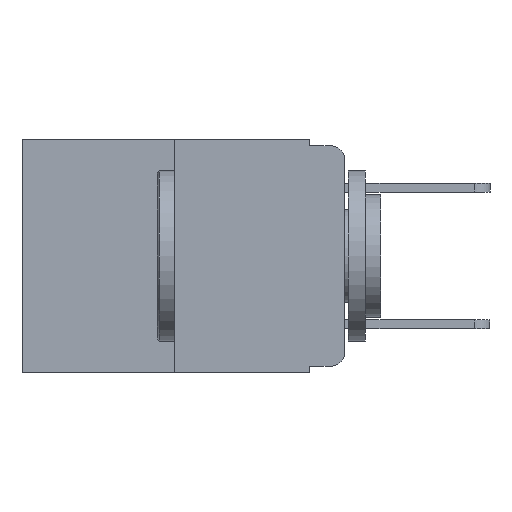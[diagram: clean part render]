
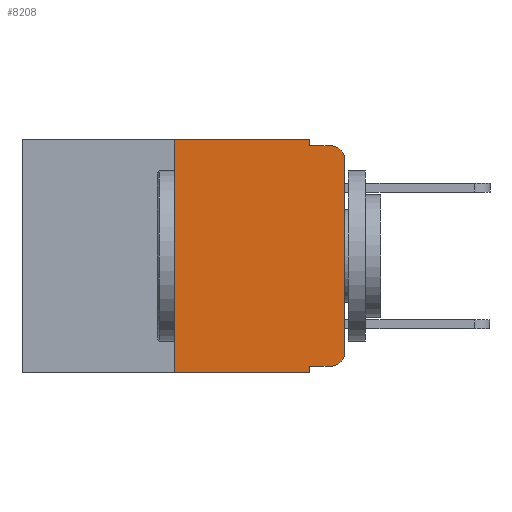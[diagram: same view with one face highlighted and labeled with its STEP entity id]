
A CAD part, left-side view. The second image highlights one B-rep face of the part: STEP entity #8208.
In plain terms, the highlighted planar face has unit normal (-1, 0, 0).
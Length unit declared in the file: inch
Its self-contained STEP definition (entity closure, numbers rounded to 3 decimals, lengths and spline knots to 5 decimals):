
#78 = ORIENTED_EDGE ( 'NONE', *, *, #8884, .T. ) ;
#179 = VECTOR ( 'NONE', #7538, 39.37008 ) ;
#377 = LINE ( 'NONE', #11194, #10634 ) ;
#400 = ORIENTED_EDGE ( 'NONE', *, *, #5301, .F. ) ;
#589 = VECTOR ( 'NONE', #1246, 39.37008 ) ;
#727 = ORIENTED_EDGE ( 'NONE', *, *, #4648, .F. ) ;
#831 = ORIENTED_EDGE ( 'NONE', *, *, #7722, .F. ) ;
#844 = VERTEX_POINT ( 'NONE', #8934 ) ;
#949 = CIRCLE ( 'NONE', #3947, 0.02 ) ;
#991 = LINE ( 'NONE', #10465, #589 ) ;
#995 = CARTESIAN_POINT ( 'NONE',  ( 0., 0.25, 0. ) ) ;
#1093 = VERTEX_POINT ( 'NONE', #7869 ) ;
#1246 = DIRECTION ( 'NONE',  ( 0., 0., -1. ) ) ;
#1350 = ORIENTED_EDGE ( 'NONE', *, *, #6838, .T. ) ;
#1418 = DIRECTION ( 'NONE',  ( 0., -1., 0. ) ) ;
#1528 = VECTOR ( 'NONE', #1418, 39.37008 ) ;
#1662 = ORIENTED_EDGE ( 'NONE', *, *, #7949, .F. ) ;
#1836 = CARTESIAN_POINT ( 'NONE',  ( 0., 0.25, -0.343 ) ) ;
#1956 = VERTEX_POINT ( 'NONE', #995 ) ;
#2018 = CIRCLE ( 'NONE', #9137, 0.02 ) ;
#2030 = VECTOR ( 'NONE', #7331, 39.37008 ) ;
#2068 = EDGE_CURVE ( 'NONE', #10869, #5049, #2018, .T. ) ;
#2095 = CARTESIAN_POINT ( 'NONE',  ( 0., 0.25, 0. ) ) ;
#2218 = DIRECTION ( 'NONE',  ( 0., 0., 1. ) ) ;
#2308 = VERTEX_POINT ( 'NONE', #6984 ) ;
#2338 = ORIENTED_EDGE ( 'NONE', *, *, #2068, .T. ) ;
#2448 = ORIENTED_EDGE ( 'NONE', *, *, #9439, .T. ) ;
#2637 = FACE_OUTER_BOUND ( 'NONE', #10825, .T. ) ;
#2736 = VERTEX_POINT ( 'NONE', #8588 ) ;
#2799 = CARTESIAN_POINT ( 'NONE',  ( 0., 0.051, 0. ) ) ;
#2853 = CARTESIAN_POINT ( 'NONE',  ( 0., 0.473, 0. ) ) ;
#3087 = VERTEX_POINT ( 'NONE', #5544 ) ;
#3395 = EDGE_CURVE ( 'NONE', #2736, #10869, #377, .T. ) ;
#3702 = CARTESIAN_POINT ( 'NONE',  ( 0., 0.02, -0.313 ) ) ;
#3719 = VERTEX_POINT ( 'NONE', #1836 ) ;
#3947 = AXIS2_PLACEMENT_3D ( 'NONE', #4903, #10981, #5855 ) ;
#4031 = EDGE_CURVE ( 'NONE', #2736, #2308, #991, .T. ) ;
#4080 = ORIENTED_EDGE ( 'NONE', *, *, #4031, .F. ) ;
#4096 = DIRECTION ( 'NONE',  ( 0., 0., -1. ) ) ;
#4201 = AXIS2_PLACEMENT_3D ( 'NONE', #11030, #4991, #11054 ) ;
#4255 = CARTESIAN_POINT ( 'NONE',  ( 0., 0.051, 0. ) ) ;
#4440 = VECTOR ( 'NONE', #2218, 39.37008 ) ;
#4560 = VECTOR ( 'NONE', #7439, 39.37008 ) ;
#4590 = LINE ( 'NONE', #6442, #2030 ) ;
#4648 = EDGE_CURVE ( 'NONE', #3719, #1956, #7183, .T. ) ;
#4903 = CARTESIAN_POINT ( 'NONE',  ( 0., 0.02, -0.03 ) ) ;
#4991 = DIRECTION ( 'NONE',  ( 1., 0., 0. ) ) ;
#5049 = VERTEX_POINT ( 'NONE', #5319 ) ;
#5301 = EDGE_CURVE ( 'NONE', #10631, #1093, #7029, .T. ) ;
#5319 = CARTESIAN_POINT ( 'NONE',  ( 0., 0., -0.313 ) ) ;
#5544 = CARTESIAN_POINT ( 'NONE',  ( 0., 0.02, -0.01 ) ) ;
#5660 = LINE ( 'NONE', #2853, #179 ) ;
#5855 = DIRECTION ( 'NONE',  ( 0., 0., -1. ) ) ;
#6178 = LINE ( 'NONE', #9025, #8261 ) ;
#6442 = CARTESIAN_POINT ( 'NONE',  ( 0., 0.051, -0.01 ) ) ;
#6838 = EDGE_CURVE ( 'NONE', #3719, #2308, #8984, .T. ) ;
#6984 = CARTESIAN_POINT ( 'NONE',  ( 0., 0.051, -0.343 ) ) ;
#7029 = LINE ( 'NONE', #2799, #4560 ) ;
#7183 = LINE ( 'NONE', #2095, #4440 ) ;
#7331 = DIRECTION ( 'NONE',  ( 0., -1., 0. ) ) ;
#7439 = DIRECTION ( 'NONE',  ( 0., 0., -1. ) ) ;
#7509 = ORIENTED_EDGE ( 'NONE', *, *, #3395, .T. ) ;
#7538 = DIRECTION ( 'NONE',  ( 0., -1., 0. ) ) ;
#7722 = EDGE_CURVE ( 'NONE', #1093, #3087, #4590, .T. ) ;
#7869 = CARTESIAN_POINT ( 'NONE',  ( 0., 0.051, -0.01 ) ) ;
#7949 = EDGE_CURVE ( 'NONE', #1956, #10631, #5660, .T. ) ;
#8040 = CARTESIAN_POINT ( 'NONE',  ( 0., 0.473, -0.343 ) ) ;
#8208 = ADVANCED_FACE ( 'NONE', ( #2637 ), #10225, .F. ) ;
#8261 = VECTOR ( 'NONE', #9851, 39.37008 ) ;
#8285 = DIRECTION ( 'NONE',  ( -1., 0., 0. ) ) ;
#8322 = CARTESIAN_POINT ( 'NONE',  ( 0., 0.02, -0.333 ) ) ;
#8588 = CARTESIAN_POINT ( 'NONE',  ( 0., 0.051, -0.333 ) ) ;
#8884 = EDGE_CURVE ( 'NONE', #844, #3087, #949, .T. ) ;
#8934 = CARTESIAN_POINT ( 'NONE',  ( 0., 0., -0.03 ) ) ;
#8984 = LINE ( 'NONE', #8040, #1528 ) ;
#9025 = CARTESIAN_POINT ( 'NONE',  ( 0., 0., 0. ) ) ;
#9137 = AXIS2_PLACEMENT_3D ( 'NONE', #3702, #8285, #4096 ) ;
#9439 = EDGE_CURVE ( 'NONE', #5049, #844, #6178, .T. ) ;
#9851 = DIRECTION ( 'NONE',  ( 0., 0., 1. ) ) ;
#10225 = PLANE ( 'NONE',  #4201 ) ;
#10465 = CARTESIAN_POINT ( 'NONE',  ( 0., 0.051, 0. ) ) ;
#10631 = VERTEX_POINT ( 'NONE', #4255 ) ;
#10634 = VECTOR ( 'NONE', #11966, 39.37008 ) ;
#10825 = EDGE_LOOP ( 'NONE', ( #2448, #78, #831, #400, #1662, #727, #1350, #4080, #7509, #2338 ) ) ;
#10869 = VERTEX_POINT ( 'NONE', #8322 ) ;
#10981 = DIRECTION ( 'NONE',  ( -1., 0., 0. ) ) ;
#11030 = CARTESIAN_POINT ( 'NONE',  ( 0., 0.473, 0. ) ) ;
#11054 = DIRECTION ( 'NONE',  ( 0., 0., -1. ) ) ;
#11194 = CARTESIAN_POINT ( 'NONE',  ( 0., 0.051, -0.333 ) ) ;
#11966 = DIRECTION ( 'NONE',  ( 0., -1., 0. ) ) ;
